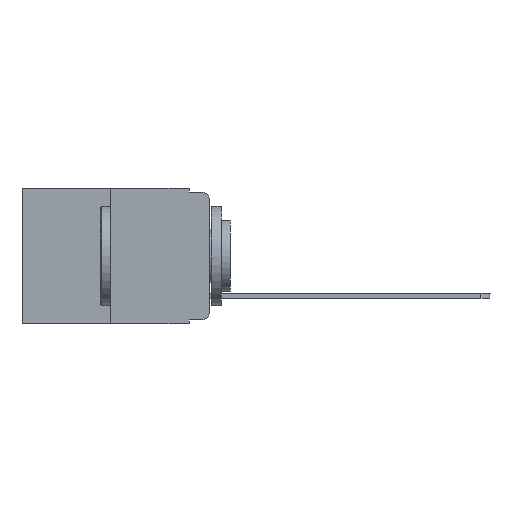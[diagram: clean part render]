
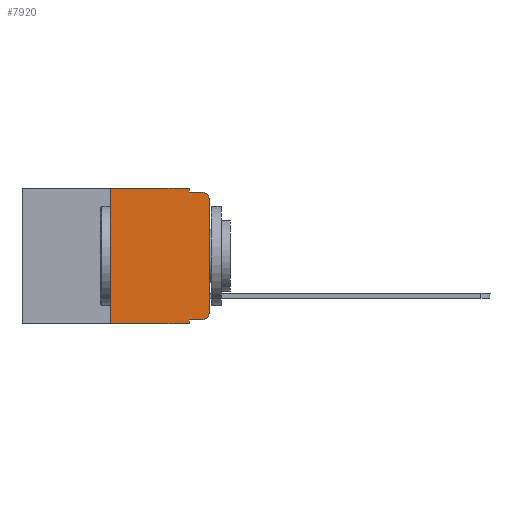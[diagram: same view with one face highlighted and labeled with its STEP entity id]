
A CAD part, left-side view. The second image highlights one B-rep face of the part: STEP entity #7920.
In plain terms, the highlighted planar face has unit normal (-1, 0, 0).
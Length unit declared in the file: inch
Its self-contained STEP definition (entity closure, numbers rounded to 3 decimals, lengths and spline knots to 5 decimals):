
#77 = CARTESIAN_POINT ( 'NONE',  ( 0., 0.473, 0. ) ) ;
#174 = VECTOR ( 'NONE', #1448, 39.37008 ) ;
#382 = DIRECTION ( 'NONE',  ( 0., 0., -1. ) ) ;
#498 = ORIENTED_EDGE ( 'NONE', *, *, #5095, .T. ) ;
#590 = LINE ( 'NONE', #5604, #5190 ) ;
#645 = AXIS2_PLACEMENT_3D ( 'NONE', #5751, #6553, #9671 ) ;
#1104 = EDGE_CURVE ( 'NONE', #2263, #9919, #4228, .T. ) ;
#1112 = ORIENTED_EDGE ( 'NONE', *, *, #1104, .T. ) ;
#1236 = DIRECTION ( 'NONE',  ( 1., 0., 0. ) ) ;
#1448 = DIRECTION ( 'NONE',  ( 0., 0., 1. ) ) ;
#1493 = EDGE_CURVE ( 'NONE', #4453, #2503, #10051, .T. ) ;
#1500 = ORIENTED_EDGE ( 'NONE', *, *, #1493, .F. ) ;
#1545 = VECTOR ( 'NONE', #6459, 39.37008 ) ;
#1746 = VERTEX_POINT ( 'NONE', #7403 ) ;
#1814 = LINE ( 'NONE', #77, #2452 ) ;
#1837 = EDGE_LOOP ( 'NONE', ( #498, #1112, #7730, #1500, #9528, #9024, #5165, #6410, #9524, #5663 ) ) ;
#2045 = CARTESIAN_POINT ( 'NONE',  ( 0., 0.473, 0. ) ) ;
#2263 = VERTEX_POINT ( 'NONE', #8190 ) ;
#2452 = VECTOR ( 'NONE', #3370, 39.37008 ) ;
#2494 = CARTESIAN_POINT ( 'NONE',  ( 0., 0.051, -0.01 ) ) ;
#2503 = VERTEX_POINT ( 'NONE', #8072 ) ;
#2802 = DIRECTION ( 'NONE',  ( 0., 0., -1. ) ) ;
#3055 = LINE ( 'NONE', #7044, #174 ) ;
#3070 = DIRECTION ( 'NONE',  ( 0., -1., 0. ) ) ;
#3335 = CARTESIAN_POINT ( 'NONE',  ( 0., 0.051, -0.333 ) ) ;
#3365 = EDGE_CURVE ( 'NONE', #7162, #5771, #3055, .T. ) ;
#3370 = DIRECTION ( 'NONE',  ( 0., -1., 0. ) ) ;
#3478 = CARTESIAN_POINT ( 'NONE',  ( 0., 0.02, -0.333 ) ) ;
#3550 = CARTESIAN_POINT ( 'NONE',  ( 0., 0.051, 0. ) ) ;
#4077 = EDGE_CURVE ( 'NONE', #6797, #9613, #5282, .T. ) ;
#4118 = AXIS2_PLACEMENT_3D ( 'NONE', #2045, #1236, #5438 ) ;
#4228 = CIRCLE ( 'NONE', #7493, 0.02 ) ;
#4453 = VERTEX_POINT ( 'NONE', #9727 ) ;
#4533 = EDGE_CURVE ( 'NONE', #7162, #9613, #590, .T. ) ;
#4622 = PLANE ( 'NONE',  #4118 ) ;
#5002 = EDGE_CURVE ( 'NONE', #5771, #4453, #1814, .T. ) ;
#5095 = EDGE_CURVE ( 'NONE', #1746, #2263, #8258, .T. ) ;
#5165 = ORIENTED_EDGE ( 'NONE', *, *, #4533, .T. ) ;
#5190 = VECTOR ( 'NONE', #3070, 39.37008 ) ;
#5282 = LINE ( 'NONE', #3550, #7252 ) ;
#5438 = DIRECTION ( 'NONE',  ( 0., 0., -1. ) ) ;
#5604 = CARTESIAN_POINT ( 'NONE',  ( 0., 0.473, -0.343 ) ) ;
#5663 = ORIENTED_EDGE ( 'NONE', *, *, #9321, .T. ) ;
#5672 = CARTESIAN_POINT ( 'NONE',  ( 0., 0.25, -0.343 ) ) ;
#5751 = CARTESIAN_POINT ( 'NONE',  ( 0., 0.02, -0.313 ) ) ;
#5771 = VERTEX_POINT ( 'NONE', #7921 ) ;
#6157 = DIRECTION ( 'NONE',  ( -1., 0., 0. ) ) ;
#6410 = ORIENTED_EDGE ( 'NONE', *, *, #4077, .F. ) ;
#6459 = DIRECTION ( 'NONE',  ( 0., -1., 0. ) ) ;
#6553 = DIRECTION ( 'NONE',  ( -1., 0., 0. ) ) ;
#6611 = CARTESIAN_POINT ( 'NONE',  ( 0., 0., 0. ) ) ;
#6797 = VERTEX_POINT ( 'NONE', #8247 ) ;
#7044 = CARTESIAN_POINT ( 'NONE',  ( 0., 0.25, 0. ) ) ;
#7162 = VERTEX_POINT ( 'NONE', #5672 ) ;
#7252 = VECTOR ( 'NONE', #2802, 39.37008 ) ;
#7351 = VECTOR ( 'NONE', #10586, 39.37008 ) ;
#7403 = CARTESIAN_POINT ( 'NONE',  ( 0., 0., -0.313 ) ) ;
#7493 = AXIS2_PLACEMENT_3D ( 'NONE', #8503, #6157, #382 ) ;
#7598 = EDGE_CURVE ( 'NONE', #6797, #9587, #10531, .T. ) ;
#7686 = DIRECTION ( 'NONE',  ( 0., 0., -1. ) ) ;
#7730 = ORIENTED_EDGE ( 'NONE', *, *, #8575, .F. ) ;
#7794 = FACE_OUTER_BOUND ( 'NONE', #1837, .T. ) ;
#7796 = CARTESIAN_POINT ( 'NONE',  ( 0., 0.051, 0. ) ) ;
#7920 = ADVANCED_FACE ( 'NONE', ( #7794 ), #4622, .F. ) ;
#7921 = CARTESIAN_POINT ( 'NONE',  ( 0., 0.25, 0. ) ) ;
#8072 = CARTESIAN_POINT ( 'NONE',  ( 0., 0.051, -0.01 ) ) ;
#8190 = CARTESIAN_POINT ( 'NONE',  ( 0., 0., -0.03 ) ) ;
#8247 = CARTESIAN_POINT ( 'NONE',  ( 0., 0.051, -0.333 ) ) ;
#8258 = LINE ( 'NONE', #6611, #10344 ) ;
#8348 = CARTESIAN_POINT ( 'NONE',  ( 0., 0.02, -0.01 ) ) ;
#8463 = VECTOR ( 'NONE', #7686, 39.37008 ) ;
#8503 = CARTESIAN_POINT ( 'NONE',  ( 0., 0.02, -0.03 ) ) ;
#8575 = EDGE_CURVE ( 'NONE', #2503, #9919, #9958, .T. ) ;
#9014 = DIRECTION ( 'NONE',  ( 0., 0., 1. ) ) ;
#9024 = ORIENTED_EDGE ( 'NONE', *, *, #3365, .F. ) ;
#9321 = EDGE_CURVE ( 'NONE', #9587, #1746, #9888, .T. ) ;
#9524 = ORIENTED_EDGE ( 'NONE', *, *, #7598, .T. ) ;
#9528 = ORIENTED_EDGE ( 'NONE', *, *, #5002, .F. ) ;
#9587 = VERTEX_POINT ( 'NONE', #3478 ) ;
#9613 = VERTEX_POINT ( 'NONE', #10353 ) ;
#9671 = DIRECTION ( 'NONE',  ( 0., 0., -1. ) ) ;
#9727 = CARTESIAN_POINT ( 'NONE',  ( 0., 0.051, 0. ) ) ;
#9888 = CIRCLE ( 'NONE', #645, 0.02 ) ;
#9919 = VERTEX_POINT ( 'NONE', #8348 ) ;
#9958 = LINE ( 'NONE', #2494, #7351 ) ;
#10051 = LINE ( 'NONE', #7796, #8463 ) ;
#10344 = VECTOR ( 'NONE', #9014, 39.37008 ) ;
#10353 = CARTESIAN_POINT ( 'NONE',  ( 0., 0.051, -0.343 ) ) ;
#10531 = LINE ( 'NONE', #3335, #1545 ) ;
#10586 = DIRECTION ( 'NONE',  ( 0., -1., 0. ) ) ;
